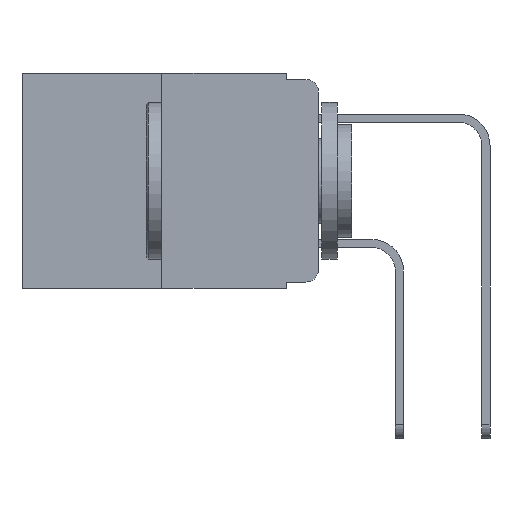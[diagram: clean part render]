
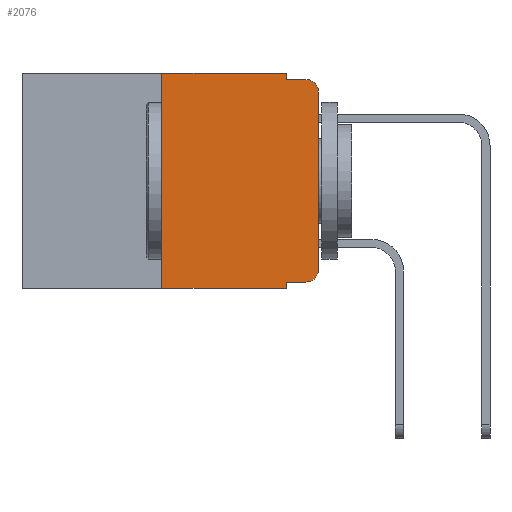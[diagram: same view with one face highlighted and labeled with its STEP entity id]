
A CAD part, left-side view. The second image highlights one B-rep face of the part: STEP entity #2076.
In plain terms, the highlighted planar face has unit normal (-1, 0, 0).
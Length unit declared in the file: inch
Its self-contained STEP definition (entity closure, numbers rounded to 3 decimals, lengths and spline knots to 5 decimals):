
#7 = FACE_OUTER_BOUND ( 'NONE', #510, .T. ) ;
#188 = CARTESIAN_POINT ( 'NONE',  ( 0., 0.051, -0.01 ) ) ;
#388 = CIRCLE ( 'NONE', #4526, 0.02 ) ;
#488 = VECTOR ( 'NONE', #10894, 39.37008 ) ;
#510 = EDGE_LOOP ( 'NONE', ( #706, #11961, #9874, #4548, #10179, #2375, #11144, #10026, #6094, #3825 ) ) ;
#706 = ORIENTED_EDGE ( 'NONE', *, *, #8324, .T. ) ;
#827 = VERTEX_POINT ( 'NONE', #5982 ) ;
#854 = VECTOR ( 'NONE', #7271, 39.37008 ) ;
#959 = DIRECTION ( 'NONE',  ( 0., 0., -1. ) ) ;
#1021 = LINE ( 'NONE', #12785, #9150 ) ;
#1243 = DIRECTION ( 'NONE',  ( 0., -1., 0. ) ) ;
#1273 = CARTESIAN_POINT ( 'NONE',  ( 0., 0.051, -0.333 ) ) ;
#1428 = DIRECTION ( 'NONE',  ( 0., 0., -1. ) ) ;
#1717 = LINE ( 'NONE', #11299, #4223 ) ;
#2076 = ADVANCED_FACE ( 'NONE', ( #7 ), #8851, .F. ) ;
#2375 = ORIENTED_EDGE ( 'NONE', *, *, #12980, .F. ) ;
#2467 = VECTOR ( 'NONE', #1428, 39.37008 ) ;
#2513 = CARTESIAN_POINT ( 'NONE',  ( 0., 0.02, -0.03 ) ) ;
#2946 = CARTESIAN_POINT ( 'NONE',  ( 0., 0.02, -0.333 ) ) ;
#3074 = AXIS2_PLACEMENT_3D ( 'NONE', #13509, #7266, #959 ) ;
#3344 = LINE ( 'NONE', #8776, #488 ) ;
#3610 = DIRECTION ( 'NONE',  ( 0., 0., -1. ) ) ;
#3825 = ORIENTED_EDGE ( 'NONE', *, *, #6799, .T. ) ;
#3933 = DIRECTION ( 'NONE',  ( 0., 0., -1. ) ) ;
#4165 = CARTESIAN_POINT ( 'NONE',  ( 0., 0.25, -0.343 ) ) ;
#4223 = VECTOR ( 'NONE', #3933, 39.37008 ) ;
#4526 = AXIS2_PLACEMENT_3D ( 'NONE', #2513, #9957, #3610 ) ;
#4548 = ORIENTED_EDGE ( 'NONE', *, *, #4701, .F. ) ;
#4701 = EDGE_CURVE ( 'NONE', #9599, #10311, #8925, .T. ) ;
#4708 = AXIS2_PLACEMENT_3D ( 'NONE', #5029, #7628, #7599 ) ;
#4827 = LINE ( 'NONE', #7129, #5148 ) ;
#4897 = VECTOR ( 'NONE', #9508, 39.37008 ) ;
#5029 = CARTESIAN_POINT ( 'NONE',  ( 0., 0.473, 0. ) ) ;
#5148 = VECTOR ( 'NONE', #8228, 39.37008 ) ;
#5228 = CARTESIAN_POINT ( 'NONE',  ( 0., 0.051, -0.01 ) ) ;
#5331 = VERTEX_POINT ( 'NONE', #5623 ) ;
#5623 = CARTESIAN_POINT ( 'NONE',  ( 0., 0., -0.03 ) ) ;
#5650 = DIRECTION ( 'NONE',  ( 0., 0., 1. ) ) ;
#5863 = CIRCLE ( 'NONE', #3074, 0.02 ) ;
#5982 = CARTESIAN_POINT ( 'NONE',  ( 0., 0., -0.313 ) ) ;
#6094 = ORIENTED_EDGE ( 'NONE', *, *, #12646, .T. ) ;
#6302 = VERTEX_POINT ( 'NONE', #6400 ) ;
#6400 = CARTESIAN_POINT ( 'NONE',  ( 0., 0.25, 0. ) ) ;
#6799 = EDGE_CURVE ( 'NONE', #10696, #827, #5863, .T. ) ;
#6880 = EDGE_CURVE ( 'NONE', #6302, #9599, #7330, .T. ) ;
#7129 = CARTESIAN_POINT ( 'NONE',  ( 0., 0.25, 0. ) ) ;
#7218 = LINE ( 'NONE', #11971, #10089 ) ;
#7266 = DIRECTION ( 'NONE',  ( -1., 0., 0. ) ) ;
#7271 = DIRECTION ( 'NONE',  ( 0., -1., 0. ) ) ;
#7330 = LINE ( 'NONE', #10593, #4897 ) ;
#7358 = EDGE_CURVE ( 'NONE', #13255, #12717, #1717, .T. ) ;
#7423 = VERTEX_POINT ( 'NONE', #8268 ) ;
#7466 = CARTESIAN_POINT ( 'NONE',  ( 0., 0.051, 0. ) ) ;
#7599 = DIRECTION ( 'NONE',  ( 0., 0., -1. ) ) ;
#7628 = DIRECTION ( 'NONE',  ( 1., 0., 0. ) ) ;
#7759 = CARTESIAN_POINT ( 'NONE',  ( 0., 0.051, 0. ) ) ;
#8228 = DIRECTION ( 'NONE',  ( 0., 0., 1. ) ) ;
#8268 = CARTESIAN_POINT ( 'NONE',  ( 0., 0.02, -0.01 ) ) ;
#8324 = EDGE_CURVE ( 'NONE', #827, #5331, #7218, .T. ) ;
#8776 = CARTESIAN_POINT ( 'NONE',  ( 0., 0.473, -0.343 ) ) ;
#8793 = CARTESIAN_POINT ( 'NONE',  ( 0., 0.051, -0.343 ) ) ;
#8851 = PLANE ( 'NONE',  #4708 ) ;
#8925 = LINE ( 'NONE', #7759, #2467 ) ;
#9150 = VECTOR ( 'NONE', #1243, 39.37008 ) ;
#9508 = DIRECTION ( 'NONE',  ( 0., -1., 0. ) ) ;
#9599 = VERTEX_POINT ( 'NONE', #7466 ) ;
#9665 = LINE ( 'NONE', #5228, #854 ) ;
#9874 = ORIENTED_EDGE ( 'NONE', *, *, #12508, .F. ) ;
#9957 = DIRECTION ( 'NONE',  ( -1., 0., 0. ) ) ;
#10026 = ORIENTED_EDGE ( 'NONE', *, *, #7358, .F. ) ;
#10089 = VECTOR ( 'NONE', #5650, 39.37008 ) ;
#10115 = VERTEX_POINT ( 'NONE', #4165 ) ;
#10179 = ORIENTED_EDGE ( 'NONE', *, *, #6880, .F. ) ;
#10311 = VERTEX_POINT ( 'NONE', #188 ) ;
#10451 = EDGE_CURVE ( 'NONE', #5331, #7423, #388, .T. ) ;
#10593 = CARTESIAN_POINT ( 'NONE',  ( 0., 0.473, 0. ) ) ;
#10696 = VERTEX_POINT ( 'NONE', #2946 ) ;
#10894 = DIRECTION ( 'NONE',  ( 0., -1., 0. ) ) ;
#11144 = ORIENTED_EDGE ( 'NONE', *, *, #13328, .T. ) ;
#11299 = CARTESIAN_POINT ( 'NONE',  ( 0., 0.051, 0. ) ) ;
#11961 = ORIENTED_EDGE ( 'NONE', *, *, #10451, .T. ) ;
#11971 = CARTESIAN_POINT ( 'NONE',  ( 0., 0., 0. ) ) ;
#12508 = EDGE_CURVE ( 'NONE', #10311, #7423, #9665, .T. ) ;
#12646 = EDGE_CURVE ( 'NONE', #13255, #10696, #1021, .T. ) ;
#12717 = VERTEX_POINT ( 'NONE', #8793 ) ;
#12785 = CARTESIAN_POINT ( 'NONE',  ( 0., 0.051, -0.333 ) ) ;
#12980 = EDGE_CURVE ( 'NONE', #10115, #6302, #4827, .T. ) ;
#13255 = VERTEX_POINT ( 'NONE', #1273 ) ;
#13328 = EDGE_CURVE ( 'NONE', #10115, #12717, #3344, .T. ) ;
#13509 = CARTESIAN_POINT ( 'NONE',  ( 0., 0.02, -0.313 ) ) ;
